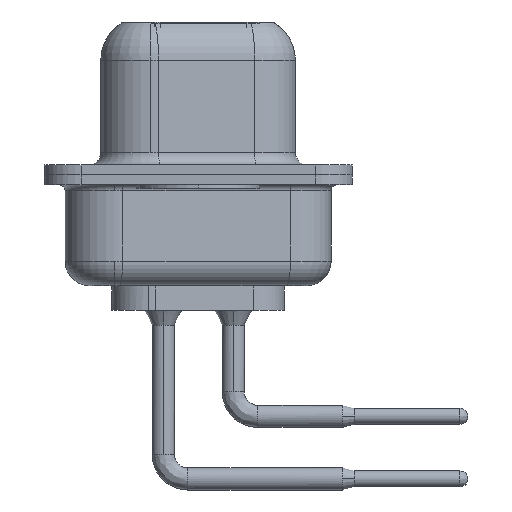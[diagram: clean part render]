
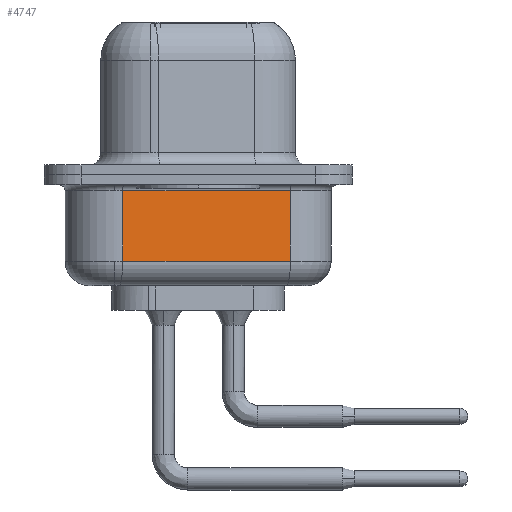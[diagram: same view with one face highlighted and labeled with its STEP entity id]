
A CAD part, left-side view. The second image highlights one B-rep face of the part: STEP entity #4747.
In plain terms, the highlighted planar face has unit normal (-0.985, -0.174, 0).
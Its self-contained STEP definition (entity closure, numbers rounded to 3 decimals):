
#942 = CARTESIAN_POINT ( 'NONE',  ( 4.054, -3.747, -3.5 ) ) ;
#1013 = VECTOR ( 'NONE', #7039, 1000. ) ;
#1180 = FACE_OUTER_BOUND ( 'NONE', #16772, .T. ) ;
#2447 = VECTOR ( 'NONE', #12295, 1000. ) ;
#3734 = DIRECTION ( 'NONE',  ( -0.174, 0.985, 0. ) ) ;
#3881 = DIRECTION ( 'NONE',  ( 0.174, -0.985, 0. ) ) ;
#4747 = ADVANCED_FACE ( 'NONE', ( #1180 ), #5311, .F. ) ;
#5311 = PLANE ( 'NONE',  #17983 ) ;
#5517 = CARTESIAN_POINT ( 'NONE',  ( 2.855, 3.053, -0.65 ) ) ;
#7039 = DIRECTION ( 'NONE',  ( 0., 0., 1. ) ) ;
#7431 = VECTOR ( 'NONE', #3734, 1000. ) ;
#9257 = CARTESIAN_POINT ( 'NONE',  ( 2.855, 3.053, -4.5 ) ) ;
#9709 = CARTESIAN_POINT ( 'NONE',  ( 2.855, 3.053, -4.5 ) ) ;
#10710 = ORIENTED_EDGE ( 'NONE', *, *, #16330, .T. ) ;
#11761 = CARTESIAN_POINT ( 'NONE',  ( 2.855, 3.053, -3.5 ) ) ;
#12295 = DIRECTION ( 'NONE',  ( 0., 0., 1. ) ) ;
#12879 = VERTEX_POINT ( 'NONE', #942 ) ;
#13123 = CARTESIAN_POINT ( 'NONE',  ( 2.855, 3.053, -0.65 ) ) ;
#13127 = ORIENTED_EDGE ( 'NONE', *, *, #17991, .T. ) ;
#13327 = EDGE_CURVE ( 'NONE', #13374, #17397, #14558, .T. ) ;
#13374 = VERTEX_POINT ( 'NONE', #17710 ) ;
#13555 = LINE ( 'NONE', #17689, #1013 ) ;
#13607 = VECTOR ( 'NONE', #3881, 1000. ) ;
#14354 = DIRECTION ( 'NONE',  ( -0.174, 0.985, 0. ) ) ;
#14397 = ORIENTED_EDGE ( 'NONE', *, *, #19410, .F. ) ;
#14529 = VERTEX_POINT ( 'NONE', #16442 ) ;
#14558 = LINE ( 'NONE', #13123, #7431 ) ;
#15822 = DIRECTION ( 'NONE',  ( 0.985, 0.174, 0. ) ) ;
#16330 = EDGE_CURVE ( 'NONE', #14529, #12879, #17597, .T. ) ;
#16442 = CARTESIAN_POINT ( 'NONE',  ( 2.855, 3.053, -3.5 ) ) ;
#16772 = EDGE_LOOP ( 'NONE', ( #14397, #10710, #13127, #19846 ) ) ;
#17397 = VERTEX_POINT ( 'NONE', #5517 ) ;
#17597 = LINE ( 'NONE', #11761, #13607 ) ;
#17689 = CARTESIAN_POINT ( 'NONE',  ( 4.054, -3.747, -4.5 ) ) ;
#17710 = CARTESIAN_POINT ( 'NONE',  ( 4.054, -3.747, -0.65 ) ) ;
#17983 = AXIS2_PLACEMENT_3D ( 'NONE', #9709, #15822, #14354 ) ;
#17991 = EDGE_CURVE ( 'NONE', #12879, #13374, #13555, .T. ) ;
#18934 = LINE ( 'NONE', #9257, #2447 ) ;
#19410 = EDGE_CURVE ( 'NONE', #14529, #17397, #18934, .T. ) ;
#19846 = ORIENTED_EDGE ( 'NONE', *, *, #13327, .T. ) ;
